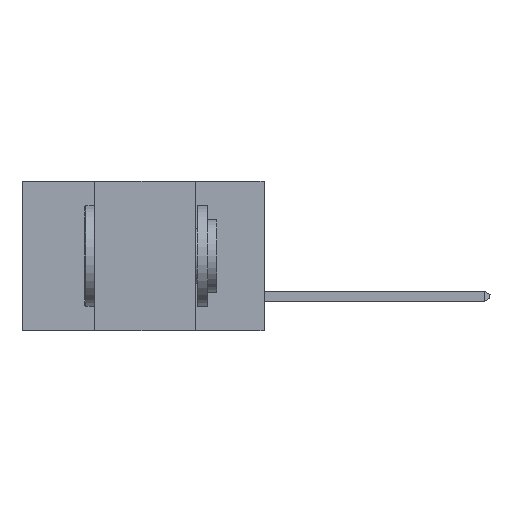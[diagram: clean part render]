
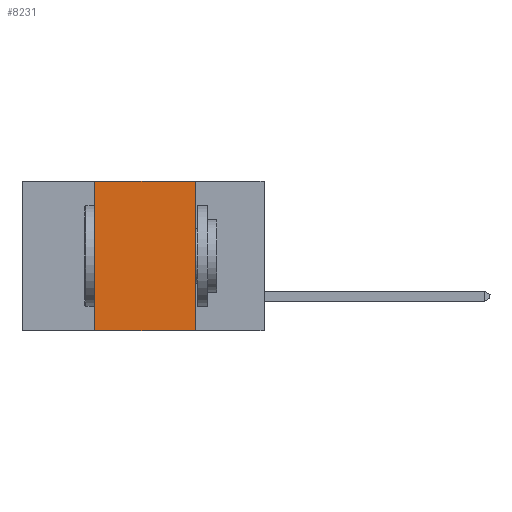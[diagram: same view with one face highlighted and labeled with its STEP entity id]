
A CAD part, left-side view. The second image highlights one B-rep face of the part: STEP entity #8231.
In plain terms, the highlighted planar face has unit normal (-1, 0, 0).
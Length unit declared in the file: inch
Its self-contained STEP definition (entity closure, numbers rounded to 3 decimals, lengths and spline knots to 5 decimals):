
#34 = DIRECTION ( 'NONE',  ( 0., 0., -1. ) ) ;
#2388 = EDGE_CURVE ( 'NONE', #8457, #13936, #7670, .T. ) ;
#2472 = VECTOR ( 'NONE', #6850, 39.37008 ) ;
#2950 = CARTESIAN_POINT ( 'NONE',  ( 0., 0.17, 0. ) ) ;
#3166 = DIRECTION ( 'NONE',  ( 0., 0., 1. ) ) ;
#3830 = PLANE ( 'NONE',  #7176 ) ;
#3896 = CARTESIAN_POINT ( 'NONE',  ( 0., 0.6, 0. ) ) ;
#4535 = LINE ( 'NONE', #2950, #18373 ) ;
#5024 = EDGE_CURVE ( 'NONE', #13921, #17597, #5716, .T. ) ;
#5050 = EDGE_CURVE ( 'NONE', #8457, #13921, #7564, .T. ) ;
#5389 = DIRECTION ( 'NONE',  ( 0., 0., -1. ) ) ;
#5716 = LINE ( 'NONE', #13039, #2472 ) ;
#6083 = CARTESIAN_POINT ( 'NONE',  ( 0., 0.42, 0. ) ) ;
#6282 = ORIENTED_EDGE ( 'NONE', *, *, #5050, .F. ) ;
#6850 = DIRECTION ( 'NONE',  ( 0., -1., 0. ) ) ;
#7099 = CARTESIAN_POINT ( 'NONE',  ( 0., 0.17, 0. ) ) ;
#7176 = AXIS2_PLACEMENT_3D ( 'NONE', #3896, #14164, #5389 ) ;
#7564 = LINE ( 'NONE', #9063, #11017 ) ;
#7670 = LINE ( 'NONE', #12660, #13671 ) ;
#8231 = ADVANCED_FACE ( 'NONE', ( #12271 ), #3830, .F. ) ;
#8457 = VERTEX_POINT ( 'NONE', #18801 ) ;
#9063 = CARTESIAN_POINT ( 'NONE',  ( 0., 0.42, 0. ) ) ;
#9898 = ORIENTED_EDGE ( 'NONE', *, *, #2388, .T. ) ;
#10442 = EDGE_LOOP ( 'NONE', ( #16600, #12446, #6282, #9898 ) ) ;
#10881 = EDGE_CURVE ( 'NONE', #17597, #13936, #4535, .T. ) ;
#11017 = VECTOR ( 'NONE', #3166, 39.37008 ) ;
#12271 = FACE_OUTER_BOUND ( 'NONE', #10442, .T. ) ;
#12446 = ORIENTED_EDGE ( 'NONE', *, *, #5024, .F. ) ;
#12660 = CARTESIAN_POINT ( 'NONE',  ( 0., 0.6, -0.37 ) ) ;
#13039 = CARTESIAN_POINT ( 'NONE',  ( 0., 0.6, 0. ) ) ;
#13671 = VECTOR ( 'NONE', #17487, 39.37008 ) ;
#13921 = VERTEX_POINT ( 'NONE', #6083 ) ;
#13936 = VERTEX_POINT ( 'NONE', #16375 ) ;
#14164 = DIRECTION ( 'NONE',  ( 1., 0., 0. ) ) ;
#16375 = CARTESIAN_POINT ( 'NONE',  ( 0., 0.17, -0.37 ) ) ;
#16600 = ORIENTED_EDGE ( 'NONE', *, *, #10881, .F. ) ;
#17487 = DIRECTION ( 'NONE',  ( 0., -1., 0. ) ) ;
#17597 = VERTEX_POINT ( 'NONE', #7099 ) ;
#18373 = VECTOR ( 'NONE', #34, 39.37008 ) ;
#18801 = CARTESIAN_POINT ( 'NONE',  ( 0., 0.42, -0.37 ) ) ;
